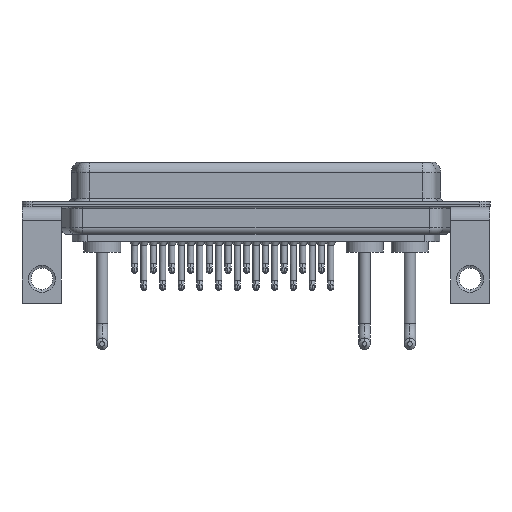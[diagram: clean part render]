
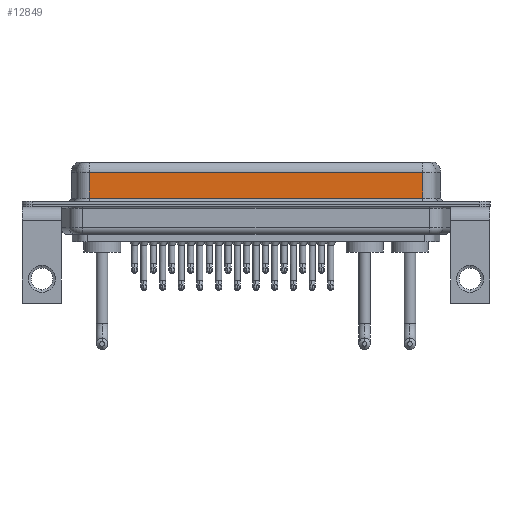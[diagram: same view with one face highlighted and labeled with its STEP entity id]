
A CAD part, front view. The second image highlights one B-rep face of the part: STEP entity #12849.
In plain terms, the highlighted planar face has unit normal (0, -1, 0).
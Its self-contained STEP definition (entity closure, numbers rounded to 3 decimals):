
#20 = ORIENTED_EDGE ( 'NONE', *, *, #13150, .T. ) ;
#567 = CARTESIAN_POINT ( 'NONE',  ( 7.038, -3.95, 6.4 ) ) ;
#1889 = ORIENTED_EDGE ( 'NONE', *, *, #15193, .F. ) ;
#2487 = CARTESIAN_POINT ( 'NONE',  ( 56.462, -3.95, 0.9 ) ) ;
#3959 = DIRECTION ( 'NONE',  ( 0., 0., 1. ) ) ;
#5416 = LINE ( 'NONE', #12658, #19707 ) ;
#5682 = VERTEX_POINT ( 'NONE', #13027 ) ;
#5947 = DIRECTION ( 'NONE',  ( 0., 1., 0. ) ) ;
#6278 = DIRECTION ( 'NONE',  ( 0., 0., -1. ) ) ;
#7452 = ORIENTED_EDGE ( 'NONE', *, *, #12192, .T. ) ;
#8020 = LINE ( 'NONE', #567, #9222 ) ;
#8785 = CARTESIAN_POINT ( 'NONE',  ( 56.462, -3.95, 4.65 ) ) ;
#9222 = VECTOR ( 'NONE', #6278, 1000. ) ;
#9411 = FACE_OUTER_BOUND ( 'NONE', #23124, .T. ) ;
#9540 = PLANE ( 'NONE',  #20385 ) ;
#10836 = VECTOR ( 'NONE', #20391, 1000. ) ;
#11220 = VERTEX_POINT ( 'NONE', #2487 ) ;
#12192 = EDGE_CURVE ( 'NONE', #23921, #5682, #8020, .T. ) ;
#12658 = CARTESIAN_POINT ( 'NONE',  ( 56.462, -3.95, 6.4 ) ) ;
#12849 = ADVANCED_FACE ( 'NONE', ( #9411 ), #9540, .F. ) ;
#13027 = CARTESIAN_POINT ( 'NONE',  ( 7.038, -3.95, 0.9 ) ) ;
#13150 = EDGE_CURVE ( 'NONE', #5682, #11220, #24450, .T. ) ;
#13984 = ORIENTED_EDGE ( 'NONE', *, *, #17820, .T. ) ;
#14745 = CARTESIAN_POINT ( 'NONE',  ( 56.462, -3.95, 0.9 ) ) ;
#14864 = DIRECTION ( 'NONE',  ( 0., 0., -1. ) ) ;
#15193 = EDGE_CURVE ( 'NONE', #19544, #11220, #5416, .T. ) ;
#16534 = LINE ( 'NONE', #16663, #10836 ) ;
#16663 = CARTESIAN_POINT ( 'NONE',  ( 56.462, -3.95, 4.65 ) ) ;
#17820 = EDGE_CURVE ( 'NONE', #19544, #23921, #16534, .T. ) ;
#19130 = CARTESIAN_POINT ( 'NONE',  ( 56.462, -3.95, 6.4 ) ) ;
#19544 = VERTEX_POINT ( 'NONE', #8785 ) ;
#19707 = VECTOR ( 'NONE', #14864, 1000. ) ;
#20385 = AXIS2_PLACEMENT_3D ( 'NONE', #19130, #5947, #3959 ) ;
#20391 = DIRECTION ( 'NONE',  ( -1., 0., 0. ) ) ;
#22067 = CARTESIAN_POINT ( 'NONE',  ( 7.038, -3.95, 4.65 ) ) ;
#22786 = VECTOR ( 'NONE', #24327, 1000. ) ;
#23124 = EDGE_LOOP ( 'NONE', ( #1889, #13984, #7452, #20 ) ) ;
#23921 = VERTEX_POINT ( 'NONE', #22067 ) ;
#24327 = DIRECTION ( 'NONE',  ( 1., 0., 0. ) ) ;
#24450 = LINE ( 'NONE', #14745, #22786 ) ;
